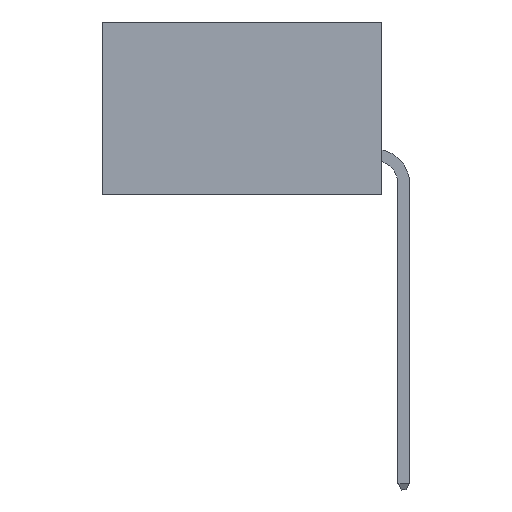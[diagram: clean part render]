
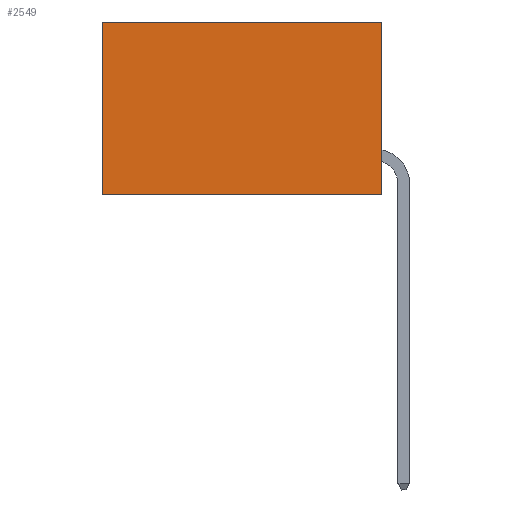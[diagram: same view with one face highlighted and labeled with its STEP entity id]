
A CAD part, left-side view. The second image highlights one B-rep face of the part: STEP entity #2549.
In plain terms, the highlighted planar face has unit normal (-1, 0, 0).
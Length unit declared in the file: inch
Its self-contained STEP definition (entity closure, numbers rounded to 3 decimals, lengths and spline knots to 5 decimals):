
#18 = VECTOR ( 'NONE', #1104, 39.37008 ) ;
#398 = EDGE_LOOP ( 'NONE', ( #6970, #883, #6357, #6487 ) ) ;
#883 = ORIENTED_EDGE ( 'NONE', *, *, #9260, .F. ) ;
#1104 = DIRECTION ( 'NONE',  ( 0., 0., -1. ) ) ;
#1476 = DIRECTION ( 'NONE',  ( 0., 1., 0. ) ) ;
#1813 = CARTESIAN_POINT ( 'NONE',  ( 0.2875, 0., -0.37 ) ) ;
#2165 = CARTESIAN_POINT ( 'NONE',  ( 0.2875, 0.6, 0. ) ) ;
#2438 = EDGE_CURVE ( 'NONE', #6737, #13811, #9605, .T. ) ;
#2445 = DIRECTION ( 'NONE',  ( 0., 1., 0. ) ) ;
#2459 = CARTESIAN_POINT ( 'NONE',  ( 0.2875, 0., 0. ) ) ;
#2549 = ADVANCED_FACE ( 'NONE', ( #4820 ), #11068, .F. ) ;
#2969 = EDGE_CURVE ( 'NONE', #6737, #13961, #5518, .T. ) ;
#3343 = EDGE_CURVE ( 'NONE', #13961, #10036, #6567, .T. ) ;
#3603 = VECTOR ( 'NONE', #8666, 39.37008 ) ;
#4224 = CARTESIAN_POINT ( 'NONE',  ( 0.2875, 0.6, 0. ) ) ;
#4616 = DIRECTION ( 'NONE',  ( 0., 0., -1. ) ) ;
#4820 = FACE_OUTER_BOUND ( 'NONE', #398, .T. ) ;
#5406 = CARTESIAN_POINT ( 'NONE',  ( 0.2875, 0., 0. ) ) ;
#5518 = LINE ( 'NONE', #5406, #14135 ) ;
#5832 = CARTESIAN_POINT ( 'NONE',  ( 0.2875, 0., 0. ) ) ;
#6166 = VECTOR ( 'NONE', #2445, 39.37008 ) ;
#6357 = ORIENTED_EDGE ( 'NONE', *, *, #2438, .F. ) ;
#6487 = ORIENTED_EDGE ( 'NONE', *, *, #2969, .T. ) ;
#6567 = LINE ( 'NONE', #4224, #18 ) ;
#6737 = VERTEX_POINT ( 'NONE', #2459 ) ;
#6857 = AXIS2_PLACEMENT_3D ( 'NONE', #9823, #9867, #4616 ) ;
#6970 = ORIENTED_EDGE ( 'NONE', *, *, #3343, .T. ) ;
#8666 = DIRECTION ( 'NONE',  ( 0., 0., -1. ) ) ;
#9172 = LINE ( 'NONE', #13718, #6166 ) ;
#9260 = EDGE_CURVE ( 'NONE', #13811, #10036, #9172, .T. ) ;
#9605 = LINE ( 'NONE', #5832, #3603 ) ;
#9823 = CARTESIAN_POINT ( 'NONE',  ( 0.2875, 0., 0. ) ) ;
#9867 = DIRECTION ( 'NONE',  ( 1., 0., 0. ) ) ;
#10036 = VERTEX_POINT ( 'NONE', #12298 ) ;
#11068 = PLANE ( 'NONE',  #6857 ) ;
#12298 = CARTESIAN_POINT ( 'NONE',  ( 0.2875, 0.6, -0.37 ) ) ;
#13718 = CARTESIAN_POINT ( 'NONE',  ( 0.2875, 0., -0.37 ) ) ;
#13811 = VERTEX_POINT ( 'NONE', #1813 ) ;
#13961 = VERTEX_POINT ( 'NONE', #2165 ) ;
#14135 = VECTOR ( 'NONE', #1476, 39.37008 ) ;
